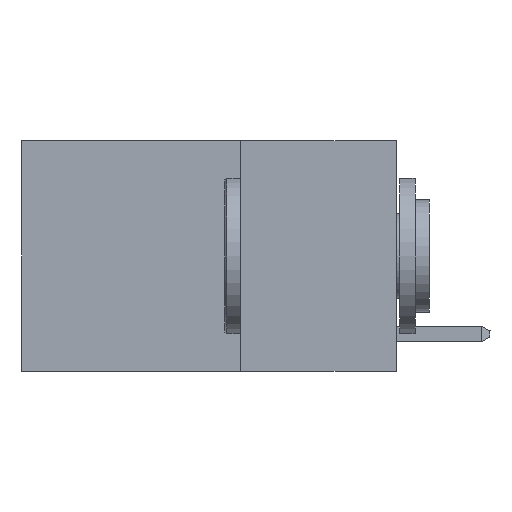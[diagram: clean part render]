
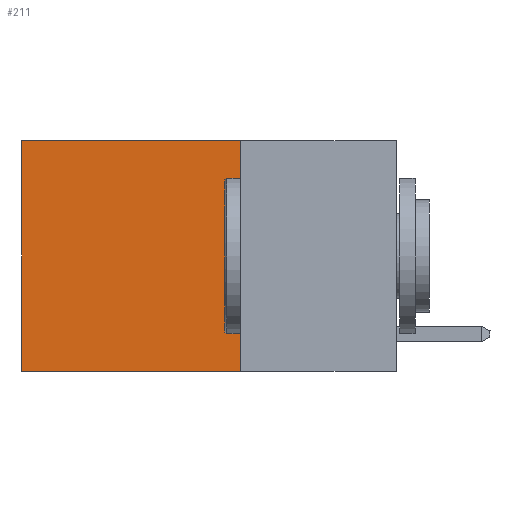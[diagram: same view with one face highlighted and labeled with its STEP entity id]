
A CAD part, left-side view. The second image highlights one B-rep face of the part: STEP entity #211.
In plain terms, the highlighted planar face has unit normal (-1, 0, 0).
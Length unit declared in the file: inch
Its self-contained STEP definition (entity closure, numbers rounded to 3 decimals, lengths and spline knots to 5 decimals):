
#91 = DIRECTION ( 'NONE',  ( 0., 0., -1. ) ) ;
#211 = ADVANCED_FACE ( 'NONE', ( #13490 ), #3556, .F. ) ;
#832 = VECTOR ( 'NONE', #11181, 39.37008 ) ;
#1666 = VECTOR ( 'NONE', #5934, 39.37008 ) ;
#2157 = CARTESIAN_POINT ( 'NONE',  ( 0.2625, 0.25, 0. ) ) ;
#2166 = CARTESIAN_POINT ( 'NONE',  ( 0.2625, 0.25, 0. ) ) ;
#3556 = PLANE ( 'NONE',  #16888 ) ;
#3915 = ORIENTED_EDGE ( 'NONE', *, *, #11204, .T. ) ;
#5042 = LINE ( 'NONE', #10704, #6277 ) ;
#5046 = CARTESIAN_POINT ( 'NONE',  ( 0.2625, 0.6, 0. ) ) ;
#5132 = VERTEX_POINT ( 'NONE', #15197 ) ;
#5519 = DIRECTION ( 'NONE',  ( 0., 1., 0. ) ) ;
#5934 = DIRECTION ( 'NONE',  ( 0., 1., 0. ) ) ;
#6277 = VECTOR ( 'NONE', #5519, 39.37008 ) ;
#6633 = CARTESIAN_POINT ( 'NONE',  ( 0.2625, 0.6, -0.37 ) ) ;
#6782 = LINE ( 'NONE', #14632, #16291 ) ;
#6816 = EDGE_CURVE ( 'NONE', #16199, #7176, #12580, .T. ) ;
#7108 = EDGE_CURVE ( 'NONE', #7428, #7176, #6782, .T. ) ;
#7176 = VERTEX_POINT ( 'NONE', #6633 ) ;
#7428 = VERTEX_POINT ( 'NONE', #5046 ) ;
#8292 = ORIENTED_EDGE ( 'NONE', *, *, #6816, .F. ) ;
#8441 = EDGE_LOOP ( 'NONE', ( #12309, #8292, #10225, #3915 ) ) ;
#10225 = ORIENTED_EDGE ( 'NONE', *, *, #14161, .F. ) ;
#10704 = CARTESIAN_POINT ( 'NONE',  ( 0.2625, 0.25, 0. ) ) ;
#11181 = DIRECTION ( 'NONE',  ( 0., 0., -1. ) ) ;
#11204 = EDGE_CURVE ( 'NONE', #5132, #7428, #5042, .T. ) ;
#11352 = CARTESIAN_POINT ( 'NONE',  ( 0.2625, 0.25, -0.37 ) ) ;
#12309 = ORIENTED_EDGE ( 'NONE', *, *, #7108, .T. ) ;
#12580 = LINE ( 'NONE', #11352, #1666 ) ;
#12670 = DIRECTION ( 'NONE',  ( 1., 0., 0. ) ) ;
#13490 = FACE_OUTER_BOUND ( 'NONE', #8441, .T. ) ;
#13745 = CARTESIAN_POINT ( 'NONE',  ( 0.2625, 0.25, -0.37 ) ) ;
#14161 = EDGE_CURVE ( 'NONE', #5132, #16199, #15460, .T. ) ;
#14632 = CARTESIAN_POINT ( 'NONE',  ( 0.2625, 0.6, 0. ) ) ;
#15197 = CARTESIAN_POINT ( 'NONE',  ( 0.2625, 0.25, 0. ) ) ;
#15460 = LINE ( 'NONE', #2166, #832 ) ;
#16199 = VERTEX_POINT ( 'NONE', #13745 ) ;
#16291 = VECTOR ( 'NONE', #91, 39.37008 ) ;
#16654 = DIRECTION ( 'NONE',  ( 0., 0., -1. ) ) ;
#16888 = AXIS2_PLACEMENT_3D ( 'NONE', #2157, #12670, #16654 ) ;
